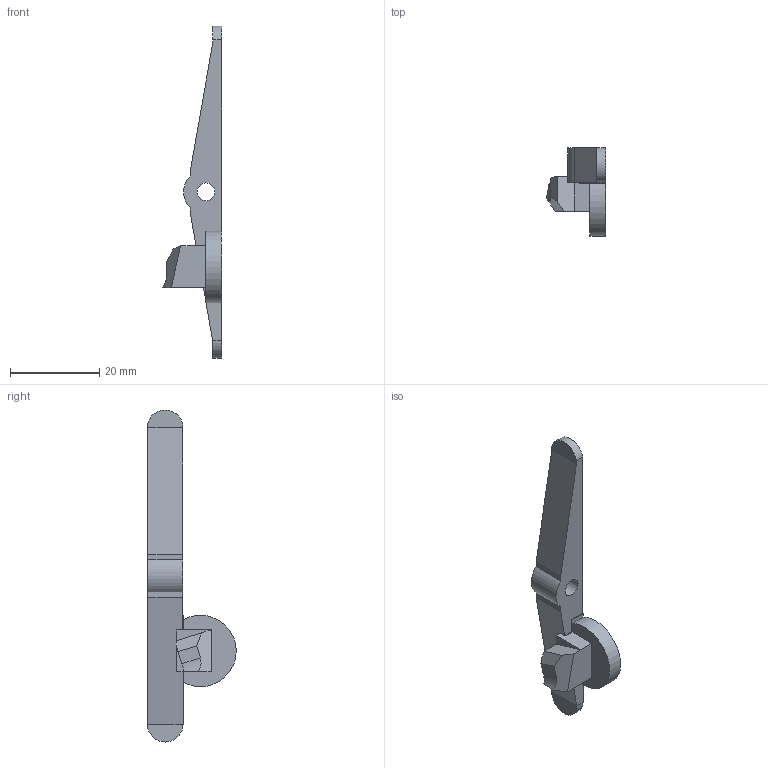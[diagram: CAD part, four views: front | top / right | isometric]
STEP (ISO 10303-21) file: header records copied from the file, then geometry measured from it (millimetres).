
FILE_DESCRIPTION(('FreeCAD Model'),'2;1');
FILE_NAME('Mag_Release_Right_V0.2A.STEP','2017-09-05T20:33:28',('Author'), (''),'Open CASCADE STEP processor 6.8','FreeCAD','Unknown');
FILE_SCHEMA(('AUTOMOTIVE_DESIGN_CC2 { 1 2 10303 214 -1 1 5 4 }'));
Length unit declared in the file: millimetre
Products named in the file (1): Pocket001
Bounding box: 13.25 x 19.81 x 74.4 mm (x, y, z)
Volume: 3665.2 mm3; surface area: 2556 mm2
Topology: 1 solids, 1 shells, 33 faces, 91 edges, 60 vertices
Faces by surface type: plane 27, cylinder 6
Full cylindrical faces by diameter (mm): 4 x1
Entity records: 2553 total; most frequent: CARTESIAN_POINT 800, DIRECTION 292, LINE 195, VECTOR 195, ORIENTED_EDGE 182, PCURVE 182, DEFINITIONAL_REPRESENTATION 182, EDGE_CURVE 91
